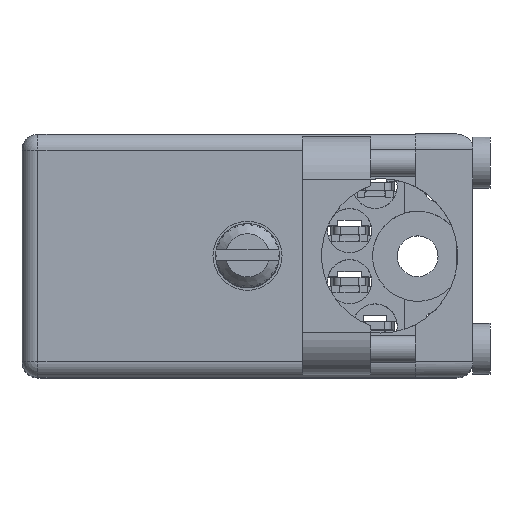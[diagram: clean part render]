
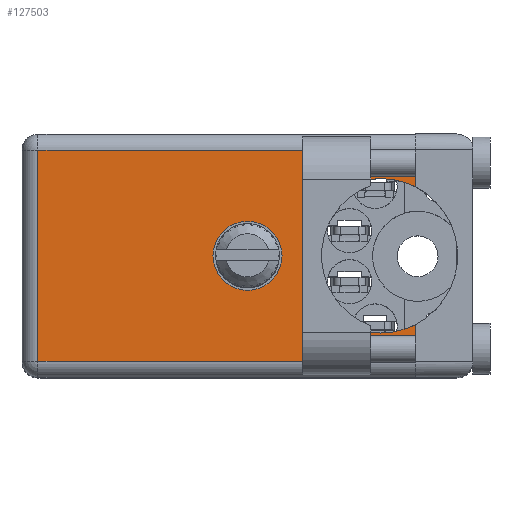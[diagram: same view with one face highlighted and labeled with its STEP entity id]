
A CAD part, top view. The second image highlights one B-rep face of the part: STEP entity #127503.
In plain terms, the highlighted face is planar.
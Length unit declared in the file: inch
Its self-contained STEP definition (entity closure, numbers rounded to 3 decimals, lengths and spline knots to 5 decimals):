
#737 = DIRECTION ( 'NONE',  ( 0., 0., 1. ) ) ;
#4074 = EDGE_CURVE ( 'NONE', #58921, #86841, #11208, .T. ) ;
#8739 = ORIENTED_EDGE ( 'NONE', *, *, #115513, .T. ) ;
#8755 = EDGE_CURVE ( 'NONE', #51954, #37223, #99891, .T. ) ;
#11098 = ORIENTED_EDGE ( 'NONE', *, *, #139629, .T. ) ;
#11208 = LINE ( 'NONE', #104192, #151252 ) ;
#16871 = ORIENTED_EDGE ( 'NONE', *, *, #62401, .F. ) ;
#19955 = DIRECTION ( 'NONE',  ( 0., 0., 1. ) ) ;
#20137 = DIRECTION ( 'NONE',  ( -1., 0., 0. ) ) ;
#22281 = VECTOR ( 'NONE', #122722, 39.37008 ) ;
#28759 = CIRCLE ( 'NONE', #36855, 0.227 ) ;
#28841 = DIRECTION ( 'NONE',  ( 1., 0., 0. ) ) ;
#29743 = DIRECTION ( 'NONE',  ( 0., 1., 0. ) ) ;
#29858 = CARTESIAN_POINT ( 'NONE',  ( -0.6155, 0.806, -0.3575 ) ) ;
#31140 = DIRECTION ( 'NONE',  ( 0., 0., 1. ) ) ;
#32004 = CARTESIAN_POINT ( 'NONE',  ( -0.6625, 0.806, -0.3575 ) ) ;
#32159 = EDGE_LOOP ( 'NONE', ( #171670, #87938 ) ) ;
#35276 = VECTOR ( 'NONE', #28841, 39.37008 ) ;
#36855 = AXIS2_PLACEMENT_3D ( 'NONE', #68218, #29743, #102784 ) ;
#37004 = VERTEX_POINT ( 'NONE', #85477 ) ;
#37170 = VERTEX_POINT ( 'NONE', #134815 ) ;
#37223 = VERTEX_POINT ( 'NONE', #131570 ) ;
#38411 = CARTESIAN_POINT ( 'NONE',  ( -0.6155, 0.806, -0.3105 ) ) ;
#39780 = DIRECTION ( 'NONE',  ( 0., 1., 0. ) ) ;
#42241 = EDGE_CURVE ( 'NONE', #37170, #86841, #140642, .T. ) ;
#43185 = ORIENTED_EDGE ( 'NONE', *, *, #8755, .F. ) ;
#47771 = CARTESIAN_POINT ( 'NONE',  ( 0.3905, 0.806, 0. ) ) ;
#51530 = AXIS2_PLACEMENT_3D ( 'NONE', #128213, #39780, #157140 ) ;
#51756 = VERTEX_POINT ( 'NONE', #38411 ) ;
#51954 = VERTEX_POINT ( 'NONE', #82411 ) ;
#55287 = CARTESIAN_POINT ( 'NONE',  ( 0.4925, 0.806, 0.3575 ) ) ;
#55727 = DIRECTION ( 'NONE',  ( 0., 1., 0. ) ) ;
#58442 = VECTOR ( 'NONE', #136842, 39.37008 ) ;
#58921 = VERTEX_POINT ( 'NONE', #183078 ) ;
#59374 = CIRCLE ( 'NONE', #117163, 0.1015 ) ;
#59765 = CARTESIAN_POINT ( 'NONE',  ( 0.3905, 0.806, -0.227 ) ) ;
#62401 = EDGE_CURVE ( 'NONE', #164242, #58921, #28759, .T. ) ;
#67181 = EDGE_CURVE ( 'NONE', #179688, #37004, #59374, .T. ) ;
#68218 = CARTESIAN_POINT ( 'NONE',  ( 0.3905, 0.806, 0. ) ) ;
#69799 = CARTESIAN_POINT ( 'NONE',  ( 0., 0.806, -0.1015 ) ) ;
#76570 = CIRCLE ( 'NONE', #122551, 0.227 ) ;
#82411 = CARTESIAN_POINT ( 'NONE',  ( 0.4925, 0.806, -0.3105 ) ) ;
#85477 = CARTESIAN_POINT ( 'NONE',  ( 0., 0.806, 0.1015 ) ) ;
#85610 = AXIS2_PLACEMENT_3D ( 'NONE', #32004, #89694, #176281 ) ;
#86841 = VERTEX_POINT ( 'NONE', #116848 ) ;
#87938 = ORIENTED_EDGE ( 'NONE', *, *, #67181, .F. ) ;
#89694 = DIRECTION ( 'NONE',  ( 0., 1., 0. ) ) ;
#94338 = DIRECTION ( 'NONE',  ( 0., 1., 0. ) ) ;
#94504 = EDGE_CURVE ( 'NONE', #132184, #164242, #115434, .T. ) ;
#99891 = LINE ( 'NONE', #55287, #168740 ) ;
#102784 = DIRECTION ( 'NONE',  ( -1., 0., 0. ) ) ;
#104181 = DIRECTION ( 'NONE',  ( -1., 0., 0. ) ) ;
#104192 = CARTESIAN_POINT ( 'NONE',  ( 0.4925, 0.806, 0.3575 ) ) ;
#105344 = ORIENTED_EDGE ( 'NONE', *, *, #94504, .F. ) ;
#109502 = LINE ( 'NONE', #138708, #22281 ) ;
#113874 = ORIENTED_EDGE ( 'NONE', *, *, #42241, .T. ) ;
#115434 = CIRCLE ( 'NONE', #174058, 0.227 ) ;
#115513 = EDGE_CURVE ( 'NONE', #51756, #37170, #115903, .T. ) ;
#115546 = CIRCLE ( 'NONE', #51530, 0.1015 ) ;
#115903 = LINE ( 'NONE', #29858, #58442 ) ;
#116848 = CARTESIAN_POINT ( 'NONE',  ( 0.4925, 0.806, 0.3105 ) ) ;
#116919 = EDGE_CURVE ( 'NONE', #37004, #179688, #115546, .T. ) ;
#117163 = AXIS2_PLACEMENT_3D ( 'NONE', #182165, #94338, #19955 ) ;
#122551 = AXIS2_PLACEMENT_3D ( 'NONE', #47771, #122744, #20137 ) ;
#122722 = DIRECTION ( 'NONE',  ( -1., 0., 0. ) ) ;
#122744 = DIRECTION ( 'NONE',  ( 0., 1., 0. ) ) ;
#123790 = ORIENTED_EDGE ( 'NONE', *, *, #4074, .F. ) ;
#127503 = ADVANCED_FACE ( 'NONE', ( #182151, #152397 ), #133288, .T. ) ;
#128213 = CARTESIAN_POINT ( 'NONE',  ( 0., 0.806, 0. ) ) ;
#131570 = CARTESIAN_POINT ( 'NONE',  ( 0.4925, 0.806, -0.20279 ) ) ;
#132184 = VERTEX_POINT ( 'NONE', #59765 ) ;
#133288 = PLANE ( 'NONE',  #85610 ) ;
#134815 = CARTESIAN_POINT ( 'NONE',  ( -0.6155, 0.806, 0.3105 ) ) ;
#136842 = DIRECTION ( 'NONE',  ( 0., 0., 1. ) ) ;
#138708 = CARTESIAN_POINT ( 'NONE',  ( -0.6625, 0.806, -0.3105 ) ) ;
#139629 = EDGE_CURVE ( 'NONE', #51954, #51756, #109502, .T. ) ;
#139748 = CARTESIAN_POINT ( 'NONE',  ( 0.3905, 0.806, 0. ) ) ;
#140642 = LINE ( 'NONE', #188465, #35276 ) ;
#149027 = EDGE_LOOP ( 'NONE', ( #43185, #11098, #8739, #113874, #123790, #16871, #105344, #172262 ) ) ;
#151252 = VECTOR ( 'NONE', #31140, 39.37008 ) ;
#152397 = FACE_BOUND ( 'NONE', #32159, .T. ) ;
#155517 = CARTESIAN_POINT ( 'NONE',  ( 0.3905, 0.806, 0.227 ) ) ;
#157140 = DIRECTION ( 'NONE',  ( 0., 0., 1. ) ) ;
#164242 = VERTEX_POINT ( 'NONE', #155517 ) ;
#168740 = VECTOR ( 'NONE', #737, 39.37008 ) ;
#169192 = EDGE_CURVE ( 'NONE', #37223, #132184, #76570, .T. ) ;
#171670 = ORIENTED_EDGE ( 'NONE', *, *, #116919, .F. ) ;
#172262 = ORIENTED_EDGE ( 'NONE', *, *, #169192, .F. ) ;
#174058 = AXIS2_PLACEMENT_3D ( 'NONE', #139748, #55727, #104181 ) ;
#176281 = DIRECTION ( 'NONE',  ( -1., 0., 0. ) ) ;
#179688 = VERTEX_POINT ( 'NONE', #69799 ) ;
#182151 = FACE_OUTER_BOUND ( 'NONE', #149027, .T. ) ;
#182165 = CARTESIAN_POINT ( 'NONE',  ( 0., 0.806, 0. ) ) ;
#183078 = CARTESIAN_POINT ( 'NONE',  ( 0.4925, 0.806, 0.20279 ) ) ;
#188465 = CARTESIAN_POINT ( 'NONE',  ( 0.4925, 0.806, 0.3105 ) ) ;
